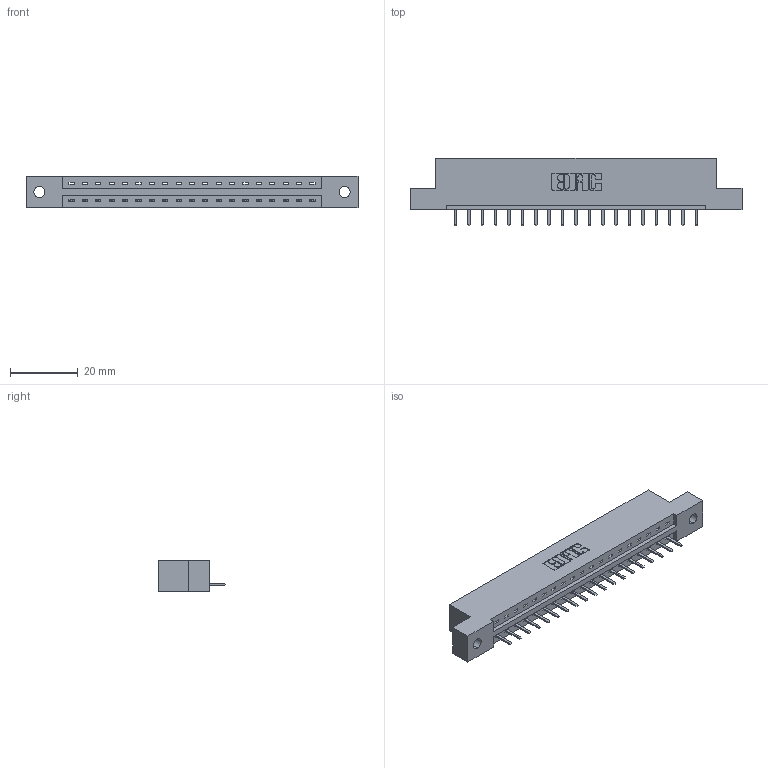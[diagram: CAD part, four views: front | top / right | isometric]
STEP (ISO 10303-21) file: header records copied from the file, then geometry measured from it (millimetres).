
FILE_DESCRIPTION (( 'STEP AP203' ), '1' );
FILE_NAME ('337-019-520-102.STEP', '2018-08-05T06:47:38', ( '' ), ( '' ), 'SwSTEP 2.0', 'SolidWorks 2016', '' );
FILE_SCHEMA (( 'CONFIG_CONTROL_DESIGN' ));
Length unit declared in the file: inch
Products named in the file (3): 337 Part_Flush Mounting Lugs - 0.128 Dia; 345-292-001_345-293-120; 337-019-520-102
Assembly tree (20 placements, depth 2):
  337-019-520-102
    337 Part_Flush Mounting Lugs - 0.128 Dia
    345-292-001_345-293-120  x19
Bounding box: 98.3 x 20.02 x 9.4 mm (x, y, z)
Volume: 9837.3 mm3; surface area: 9571.1 mm2
Topology: 20 solids, 20 shells, 1368 faces, 4035 edges, 2638 vertices
Faces by surface type: plane 982, cylinder 386
Entity records: 17215 total; most frequent: CARTESIAN_POINT 3015, ORIENTED_EDGE 2958, DIRECTION 2573, EDGE_CURVE 1479, LINE 1347, VECTOR 1347, VERTEX_POINT 982, AXIS2_PLACEMENT_3D 613
